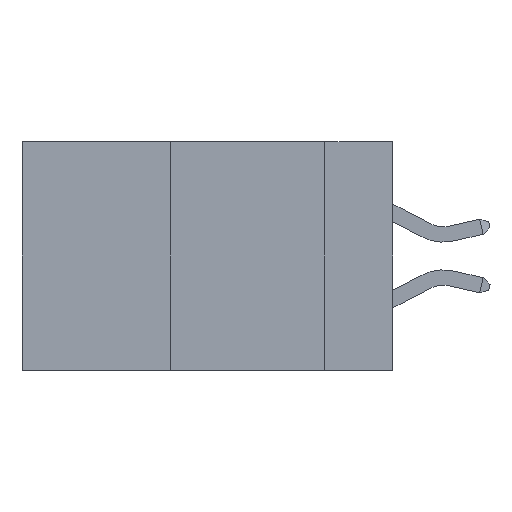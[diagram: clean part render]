
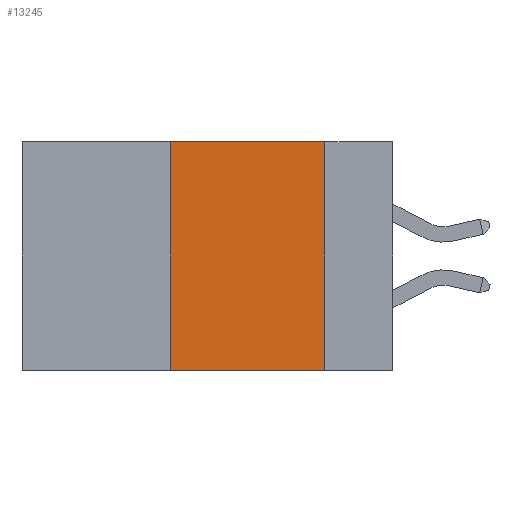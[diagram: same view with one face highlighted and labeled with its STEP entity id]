
A CAD part, left-side view. The second image highlights one B-rep face of the part: STEP entity #13245.
In plain terms, the highlighted planar face has unit normal (-1, 0, 0).
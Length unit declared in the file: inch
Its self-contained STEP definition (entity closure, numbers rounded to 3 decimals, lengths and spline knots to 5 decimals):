
#130 = VECTOR ( 'NONE', #11347, 39.37008 ) ;
#2796 = DIRECTION ( 'NONE',  ( 0., 0., 1. ) ) ;
#2918 = ORIENTED_EDGE ( 'NONE', *, *, #5790, .F. ) ;
#3286 = LINE ( 'NONE', #10333, #130 ) ;
#3288 = CARTESIAN_POINT ( 'NONE',  ( 0., 0.6, -0.37 ) ) ;
#3363 = DIRECTION ( 'NONE',  ( 0., -1., 0. ) ) ;
#3639 = EDGE_CURVE ( 'NONE', #10583, #11352, #13077, .T. ) ;
#3793 = ORIENTED_EDGE ( 'NONE', *, *, #9715, .F. ) ;
#4223 = CARTESIAN_POINT ( 'NONE',  ( 0., 0.6, 0. ) ) ;
#4333 = LINE ( 'NONE', #12874, #6819 ) ;
#4337 = EDGE_CURVE ( 'NONE', #10583, #8501, #6953, .T. ) ;
#4436 = ORIENTED_EDGE ( 'NONE', *, *, #3639, .T. ) ;
#5008 = VECTOR ( 'NONE', #3363, 39.37008 ) ;
#5035 = CARTESIAN_POINT ( 'NONE',  ( 0., 0.36, -0.37 ) ) ;
#5637 = CARTESIAN_POINT ( 'NONE',  ( 0., 0.11, 0. ) ) ;
#5745 = EDGE_LOOP ( 'NONE', ( #2918, #3793, #6416, #4436 ) ) ;
#5790 = EDGE_CURVE ( 'NONE', #12856, #11352, #3286, .T. ) ;
#5858 = DIRECTION ( 'NONE',  ( 0., -1., 0. ) ) ;
#6359 = DIRECTION ( 'NONE',  ( 1., 0., 0. ) ) ;
#6397 = FACE_OUTER_BOUND ( 'NONE', #5745, .T. ) ;
#6416 = ORIENTED_EDGE ( 'NONE', *, *, #4337, .F. ) ;
#6427 = AXIS2_PLACEMENT_3D ( 'NONE', #4223, #6359, #13360 ) ;
#6819 = VECTOR ( 'NONE', #5858, 39.37008 ) ;
#6953 = LINE ( 'NONE', #8968, #9563 ) ;
#8501 = VERTEX_POINT ( 'NONE', #12997 ) ;
#8968 = CARTESIAN_POINT ( 'NONE',  ( 0., 0.36, 0. ) ) ;
#9305 = CARTESIAN_POINT ( 'NONE',  ( 0., 0.11, -0.37 ) ) ;
#9563 = VECTOR ( 'NONE', #2796, 39.37008 ) ;
#9715 = EDGE_CURVE ( 'NONE', #8501, #12856, #4333, .T. ) ;
#10333 = CARTESIAN_POINT ( 'NONE',  ( 0., 0.11, 0. ) ) ;
#10583 = VERTEX_POINT ( 'NONE', #5035 ) ;
#11347 = DIRECTION ( 'NONE',  ( 0., 0., -1. ) ) ;
#11352 = VERTEX_POINT ( 'NONE', #9305 ) ;
#12856 = VERTEX_POINT ( 'NONE', #5637 ) ;
#12874 = CARTESIAN_POINT ( 'NONE',  ( 0., 0.6, 0. ) ) ;
#12997 = CARTESIAN_POINT ( 'NONE',  ( 0., 0.36, 0. ) ) ;
#13077 = LINE ( 'NONE', #3288, #5008 ) ;
#13245 = ADVANCED_FACE ( 'NONE', ( #6397 ), #13327, .F. ) ;
#13327 = PLANE ( 'NONE',  #6427 ) ;
#13360 = DIRECTION ( 'NONE',  ( 0., 0., -1. ) ) ;
